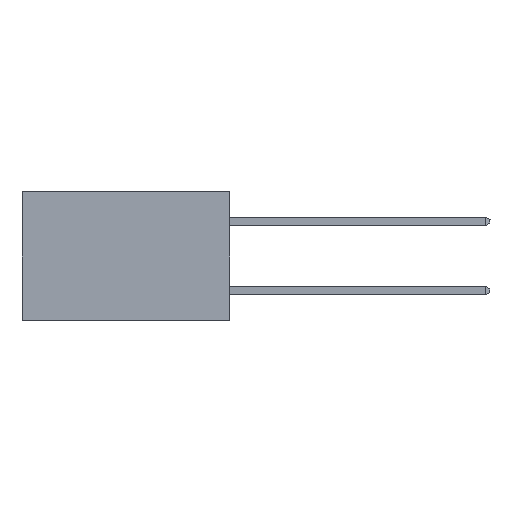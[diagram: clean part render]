
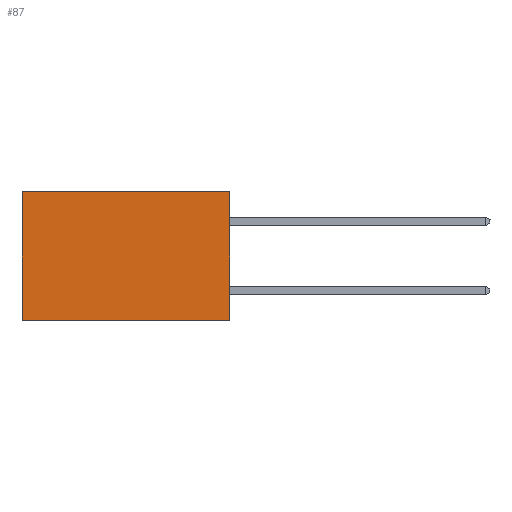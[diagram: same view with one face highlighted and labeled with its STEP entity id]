
A CAD part, left-side view. The second image highlights one B-rep face of the part: STEP entity #87.
In plain terms, the highlighted planar face has unit normal (-1, 0, 0).
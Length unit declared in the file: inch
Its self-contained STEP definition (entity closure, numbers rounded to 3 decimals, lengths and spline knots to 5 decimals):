
#87 = ADVANCED_FACE ( 'NONE', ( #15212 ), #5094, .F. ) ;
#132 = DIRECTION ( 'NONE',  ( 0., 1., 0. ) ) ;
#1076 = VECTOR ( 'NONE', #4328, 39.37008 ) ;
#1368 = CARTESIAN_POINT ( 'NONE',  ( 0.2615, 0., 0. ) ) ;
#1415 = CARTESIAN_POINT ( 'NONE',  ( 0.2615, 0.6, -0.37 ) ) ;
#1908 = EDGE_LOOP ( 'NONE', ( #7440, #3919, #12319, #16397 ) ) ;
#2000 = CARTESIAN_POINT ( 'NONE',  ( 0.2615, 0., -0.37 ) ) ;
#2649 = VECTOR ( 'NONE', #16089, 39.37008 ) ;
#3919 = ORIENTED_EDGE ( 'NONE', *, *, #16838, .F. ) ;
#4328 = DIRECTION ( 'NONE',  ( 0., 0., -1. ) ) ;
#4862 = VECTOR ( 'NONE', #13131, 39.37008 ) ;
#4972 = LINE ( 'NONE', #9023, #9370 ) ;
#5094 = PLANE ( 'NONE',  #6395 ) ;
#5576 = VERTEX_POINT ( 'NONE', #18606 ) ;
#5703 = CARTESIAN_POINT ( 'NONE',  ( 0.2615, 0.6, -0.37 ) ) ;
#5910 = LINE ( 'NONE', #8623, #4862 ) ;
#6137 = LINE ( 'NONE', #10494, #1076 ) ;
#6395 = AXIS2_PLACEMENT_3D ( 'NONE', #2000, #7891, #15309 ) ;
#7307 = LINE ( 'NONE', #1415, #2649 ) ;
#7440 = ORIENTED_EDGE ( 'NONE', *, *, #14669, .T. ) ;
#7891 = DIRECTION ( 'NONE',  ( 1., 0., 0. ) ) ;
#8623 = CARTESIAN_POINT ( 'NONE',  ( 0.2615, 0., -0.37 ) ) ;
#9023 = CARTESIAN_POINT ( 'NONE',  ( 0.2615, 0., 0. ) ) ;
#9233 = VERTEX_POINT ( 'NONE', #1368 ) ;
#9370 = VECTOR ( 'NONE', #132, 39.37008 ) ;
#10494 = CARTESIAN_POINT ( 'NONE',  ( 0.2615, 0., -0.37 ) ) ;
#12063 = EDGE_CURVE ( 'NONE', #9233, #19039, #4972, .T. ) ;
#12319 = ORIENTED_EDGE ( 'NONE', *, *, #13449, .F. ) ;
#13131 = DIRECTION ( 'NONE',  ( 0., 1., 0. ) ) ;
#13449 = EDGE_CURVE ( 'NONE', #9233, #5576, #6137, .T. ) ;
#14105 = VERTEX_POINT ( 'NONE', #5703 ) ;
#14669 = EDGE_CURVE ( 'NONE', #19039, #14105, #7307, .T. ) ;
#15212 = FACE_OUTER_BOUND ( 'NONE', #1908, .T. ) ;
#15309 = DIRECTION ( 'NONE',  ( 0., 0., -1. ) ) ;
#16089 = DIRECTION ( 'NONE',  ( 0., 0., -1. ) ) ;
#16312 = CARTESIAN_POINT ( 'NONE',  ( 0.2615, 0.6, 0. ) ) ;
#16397 = ORIENTED_EDGE ( 'NONE', *, *, #12063, .T. ) ;
#16838 = EDGE_CURVE ( 'NONE', #5576, #14105, #5910, .T. ) ;
#18606 = CARTESIAN_POINT ( 'NONE',  ( 0.2615, 0., -0.37 ) ) ;
#19039 = VERTEX_POINT ( 'NONE', #16312 ) ;
